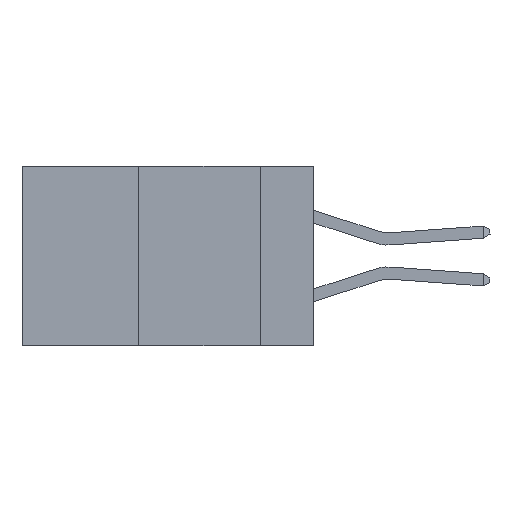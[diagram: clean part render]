
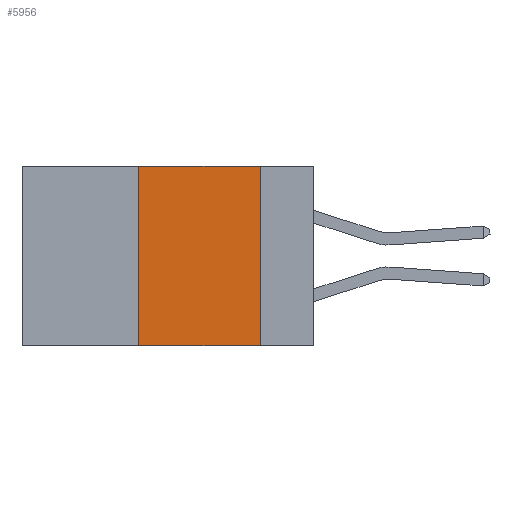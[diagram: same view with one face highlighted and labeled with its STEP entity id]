
A CAD part, left-side view. The second image highlights one B-rep face of the part: STEP entity #5956.
In plain terms, the highlighted planar face has unit normal (-1, 0, 0).
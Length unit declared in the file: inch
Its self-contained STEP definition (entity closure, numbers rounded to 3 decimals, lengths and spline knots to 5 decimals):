
#410 = CARTESIAN_POINT ( 'NONE',  ( 0., 0.36, -0.37 ) ) ;
#506 = DIRECTION ( 'NONE',  ( 0., 0., -1. ) ) ;
#691 = VERTEX_POINT ( 'NONE', #410 ) ;
#790 = AXIS2_PLACEMENT_3D ( 'NONE', #6137, #3168, #4161 ) ;
#1162 = VECTOR ( 'NONE', #506, 39.37008 ) ;
#1289 = ORIENTED_EDGE ( 'NONE', *, *, #11126, .F. ) ;
#1366 = LINE ( 'NONE', #3115, #1162 ) ;
#1455 = VERTEX_POINT ( 'NONE', #2722 ) ;
#1617 = DIRECTION ( 'NONE',  ( 0., 0., 1. ) ) ;
#2174 = DIRECTION ( 'NONE',  ( 0., -1., 0. ) ) ;
#2292 = CARTESIAN_POINT ( 'NONE',  ( 0., 0.6, -0.37 ) ) ;
#2722 = CARTESIAN_POINT ( 'NONE',  ( 0., 0.36, 0. ) ) ;
#3115 = CARTESIAN_POINT ( 'NONE',  ( 0., 0.11, 0. ) ) ;
#3168 = DIRECTION ( 'NONE',  ( 1., 0., 0. ) ) ;
#3393 = LINE ( 'NONE', #6179, #8745 ) ;
#4161 = DIRECTION ( 'NONE',  ( 0., 0., -1. ) ) ;
#4299 = ORIENTED_EDGE ( 'NONE', *, *, #4563, .F. ) ;
#4446 = CARTESIAN_POINT ( 'NONE',  ( 0., 0.11, -0.37 ) ) ;
#4563 = EDGE_CURVE ( 'NONE', #6382, #8080, #1366, .T. ) ;
#5956 = ADVANCED_FACE ( 'NONE', ( #10650 ), #11775, .F. ) ;
#6022 = EDGE_LOOP ( 'NONE', ( #4299, #1289, #7860, #9105 ) ) ;
#6137 = CARTESIAN_POINT ( 'NONE',  ( 0., 0.6, 0. ) ) ;
#6179 = CARTESIAN_POINT ( 'NONE',  ( 0., 0.6, 0. ) ) ;
#6382 = VERTEX_POINT ( 'NONE', #8357 ) ;
#7207 = VECTOR ( 'NONE', #2174, 39.37008 ) ;
#7775 = LINE ( 'NONE', #2292, #7207 ) ;
#7860 = ORIENTED_EDGE ( 'NONE', *, *, #11341, .F. ) ;
#8080 = VERTEX_POINT ( 'NONE', #4446 ) ;
#8249 = EDGE_CURVE ( 'NONE', #691, #8080, #7775, .T. ) ;
#8357 = CARTESIAN_POINT ( 'NONE',  ( 0., 0.11, 0. ) ) ;
#8745 = VECTOR ( 'NONE', #10753, 39.37008 ) ;
#9105 = ORIENTED_EDGE ( 'NONE', *, *, #8249, .T. ) ;
#9856 = CARTESIAN_POINT ( 'NONE',  ( 0., 0.36, 0. ) ) ;
#10650 = FACE_OUTER_BOUND ( 'NONE', #6022, .T. ) ;
#10753 = DIRECTION ( 'NONE',  ( 0., -1., 0. ) ) ;
#10914 = VECTOR ( 'NONE', #1617, 39.37008 ) ;
#11126 = EDGE_CURVE ( 'NONE', #1455, #6382, #3393, .T. ) ;
#11341 = EDGE_CURVE ( 'NONE', #691, #1455, #11793, .T. ) ;
#11775 = PLANE ( 'NONE',  #790 ) ;
#11793 = LINE ( 'NONE', #9856, #10914 ) ;
